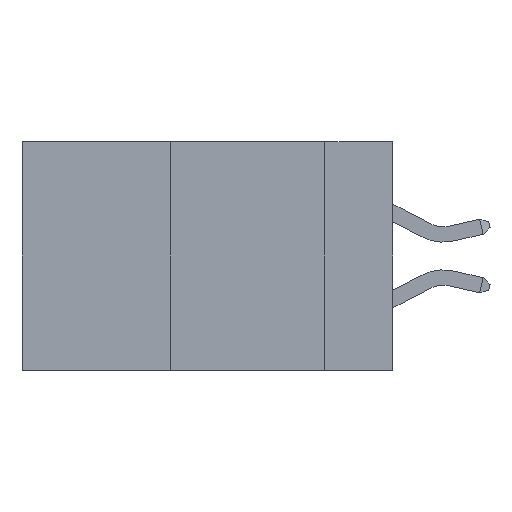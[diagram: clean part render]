
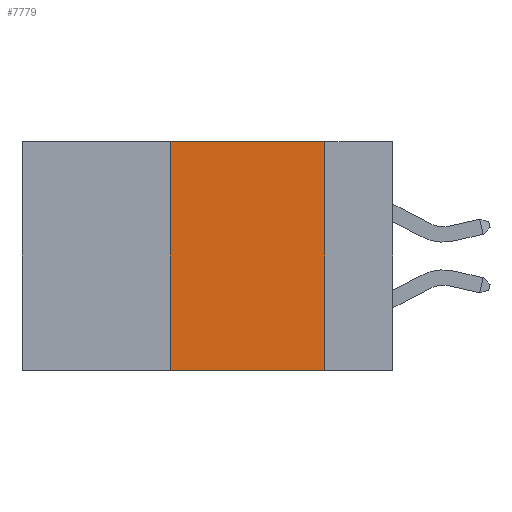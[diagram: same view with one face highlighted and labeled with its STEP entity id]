
A CAD part, left-side view. The second image highlights one B-rep face of the part: STEP entity #7779.
In plain terms, the highlighted planar face has unit normal (-1, 0, 0).
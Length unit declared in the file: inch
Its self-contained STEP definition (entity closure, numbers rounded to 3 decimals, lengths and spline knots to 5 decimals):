
#778 = VECTOR ( 'NONE', #21192, 39.37008 ) ;
#1152 = LINE ( 'NONE', #22441, #10102 ) ;
#1307 = CARTESIAN_POINT ( 'NONE',  ( 0., 0.6, 0. ) ) ;
#2470 = CARTESIAN_POINT ( 'NONE',  ( 0., 0.11, -0.37 ) ) ;
#2765 = DIRECTION ( 'NONE',  ( 1., 0., 0. ) ) ;
#2912 = ORIENTED_EDGE ( 'NONE', *, *, #8177, .T. ) ;
#4610 = CARTESIAN_POINT ( 'NONE',  ( 0., 0.36, -0.37 ) ) ;
#7732 = FACE_OUTER_BOUND ( 'NONE', #29856, .T. ) ;
#7779 = ADVANCED_FACE ( 'NONE', ( #7732 ), #8765, .F. ) ;
#8177 = EDGE_CURVE ( 'NONE', #12129, #17755, #9945, .T. ) ;
#8687 = CARTESIAN_POINT ( 'NONE',  ( 0., 0.6, -0.37 ) ) ;
#8765 = PLANE ( 'NONE',  #29142 ) ;
#9945 = LINE ( 'NONE', #8687, #35509 ) ;
#10057 = ORIENTED_EDGE ( 'NONE', *, *, #32587, .F. ) ;
#10102 = VECTOR ( 'NONE', #24942, 39.37008 ) ;
#10668 = VERTEX_POINT ( 'NONE', #27354 ) ;
#11383 = ORIENTED_EDGE ( 'NONE', *, *, #32042, .F. ) ;
#12129 = VERTEX_POINT ( 'NONE', #4610 ) ;
#14253 = DIRECTION ( 'NONE',  ( 0., 0., -1. ) ) ;
#15984 = LINE ( 'NONE', #1307, #778 ) ;
#16570 = DIRECTION ( 'NONE',  ( 0., 0., -1. ) ) ;
#17755 = VERTEX_POINT ( 'NONE', #2470 ) ;
#21192 = DIRECTION ( 'NONE',  ( 0., -1., 0. ) ) ;
#22441 = CARTESIAN_POINT ( 'NONE',  ( 0., 0.36, 0. ) ) ;
#24306 = EDGE_CURVE ( 'NONE', #30914, #10668, #15984, .T. ) ;
#24932 = VECTOR ( 'NONE', #16570, 39.37008 ) ;
#24942 = DIRECTION ( 'NONE',  ( 0., 0., 1. ) ) ;
#27354 = CARTESIAN_POINT ( 'NONE',  ( 0., 0.11, 0. ) ) ;
#27644 = LINE ( 'NONE', #33874, #24932 ) ;
#28708 = ORIENTED_EDGE ( 'NONE', *, *, #24306, .F. ) ;
#28752 = DIRECTION ( 'NONE',  ( 0., -1., 0. ) ) ;
#29142 = AXIS2_PLACEMENT_3D ( 'NONE', #37084, #2765, #14253 ) ;
#29856 = EDGE_LOOP ( 'NONE', ( #11383, #28708, #10057, #2912 ) ) ;
#30914 = VERTEX_POINT ( 'NONE', #31245 ) ;
#31245 = CARTESIAN_POINT ( 'NONE',  ( 0., 0.36, 0. ) ) ;
#32042 = EDGE_CURVE ( 'NONE', #10668, #17755, #27644, .T. ) ;
#32587 = EDGE_CURVE ( 'NONE', #12129, #30914, #1152, .T. ) ;
#33874 = CARTESIAN_POINT ( 'NONE',  ( 0., 0.11, 0. ) ) ;
#35509 = VECTOR ( 'NONE', #28752, 39.37008 ) ;
#37084 = CARTESIAN_POINT ( 'NONE',  ( 0., 0.6, 0. ) ) ;
